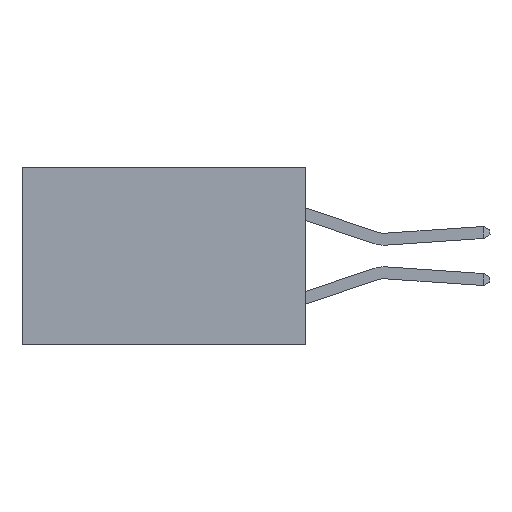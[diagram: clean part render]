
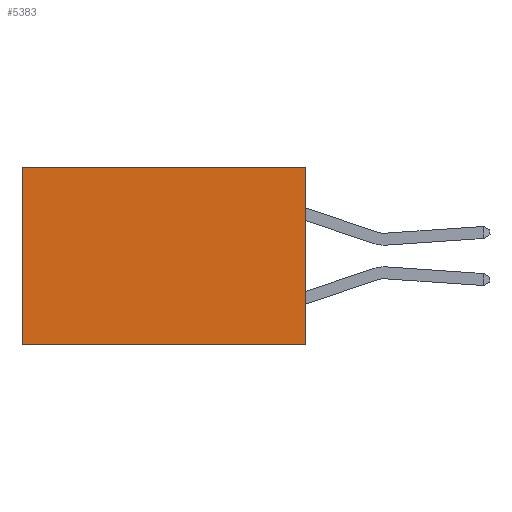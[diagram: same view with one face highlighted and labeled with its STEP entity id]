
A CAD part, left-side view. The second image highlights one B-rep face of the part: STEP entity #5383.
In plain terms, the highlighted planar face has unit normal (-1, 0, 0).
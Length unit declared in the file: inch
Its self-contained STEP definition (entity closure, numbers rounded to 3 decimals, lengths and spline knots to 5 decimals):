
#166 = CARTESIAN_POINT ( 'NONE',  ( 0.277, 0., -0.37 ) ) ;
#586 = AXIS2_PLACEMENT_3D ( 'NONE', #21802, #21506, #21502 ) ;
#1256 = CARTESIAN_POINT ( 'NONE',  ( 0.277, 0., -0.37 ) ) ;
#1367 = VERTEX_POINT ( 'NONE', #31123 ) ;
#2469 = LINE ( 'NONE', #1256, #14585 ) ;
#3230 = EDGE_CURVE ( 'NONE', #8936, #16812, #4712, .T. ) ;
#3689 = DIRECTION ( 'NONE',  ( 0., 0., -1. ) ) ;
#4712 = LINE ( 'NONE', #10325, #23725 ) ;
#4732 = VERTEX_POINT ( 'NONE', #18357 ) ;
#5383 = ADVANCED_FACE ( 'NONE', ( #29085 ), #21542, .F. ) ;
#6317 = EDGE_CURVE ( 'NONE', #1367, #4732, #18019, .T. ) ;
#6503 = LINE ( 'NONE', #9206, #24001 ) ;
#7458 = ORIENTED_EDGE ( 'NONE', *, *, #6317, .F. ) ;
#8936 = VERTEX_POINT ( 'NONE', #19341 ) ;
#9206 = CARTESIAN_POINT ( 'NONE',  ( 0.277, 0.59, -0.37 ) ) ;
#9640 = EDGE_CURVE ( 'NONE', #16812, #4732, #6503, .T. ) ;
#10325 = CARTESIAN_POINT ( 'NONE',  ( 0.277, 0., 0. ) ) ;
#10398 = DIRECTION ( 'NONE',  ( 0., 1., 0. ) ) ;
#10622 = VECTOR ( 'NONE', #30128, 39.37008 ) ;
#14585 = VECTOR ( 'NONE', #3689, 39.37008 ) ;
#16581 = DIRECTION ( 'NONE',  ( 0., 0., -1. ) ) ;
#16812 = VERTEX_POINT ( 'NONE', #28010 ) ;
#16936 = ORIENTED_EDGE ( 'NONE', *, *, #30197, .F. ) ;
#18019 = LINE ( 'NONE', #166, #10622 ) ;
#18357 = CARTESIAN_POINT ( 'NONE',  ( 0.277, 0.59, -0.37 ) ) ;
#19341 = CARTESIAN_POINT ( 'NONE',  ( 0.277, 0., 0. ) ) ;
#21502 = DIRECTION ( 'NONE',  ( 0., 0., -1. ) ) ;
#21506 = DIRECTION ( 'NONE',  ( 1., 0., 0. ) ) ;
#21542 = PLANE ( 'NONE',  #586 ) ;
#21802 = CARTESIAN_POINT ( 'NONE',  ( 0.277, 0., -0.37 ) ) ;
#22848 = ORIENTED_EDGE ( 'NONE', *, *, #3230, .T. ) ;
#23725 = VECTOR ( 'NONE', #10398, 39.37008 ) ;
#24001 = VECTOR ( 'NONE', #16581, 39.37008 ) ;
#27006 = ORIENTED_EDGE ( 'NONE', *, *, #9640, .T. ) ;
#28010 = CARTESIAN_POINT ( 'NONE',  ( 0.277, 0.59, 0. ) ) ;
#29085 = FACE_OUTER_BOUND ( 'NONE', #30041, .T. ) ;
#30041 = EDGE_LOOP ( 'NONE', ( #27006, #7458, #16936, #22848 ) ) ;
#30128 = DIRECTION ( 'NONE',  ( 0., 1., 0. ) ) ;
#30197 = EDGE_CURVE ( 'NONE', #8936, #1367, #2469, .T. ) ;
#31123 = CARTESIAN_POINT ( 'NONE',  ( 0.277, 0., -0.37 ) ) ;
